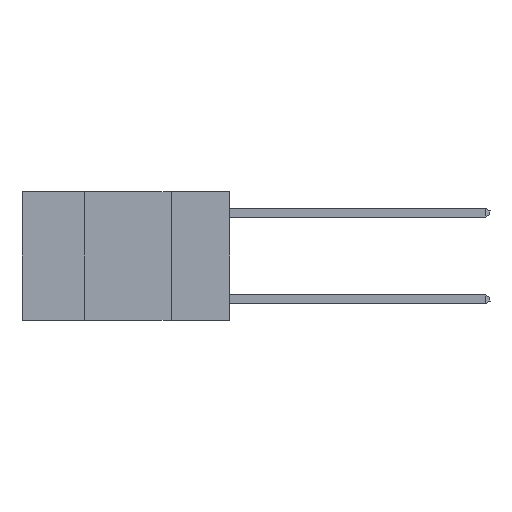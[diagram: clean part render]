
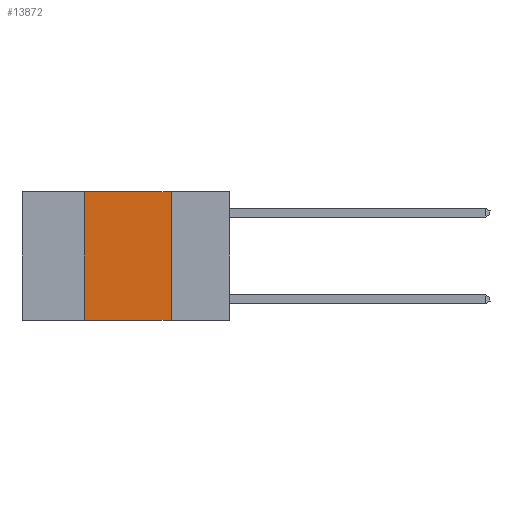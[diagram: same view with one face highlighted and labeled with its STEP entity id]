
A CAD part, left-side view. The second image highlights one B-rep face of the part: STEP entity #13872.
In plain terms, the highlighted planar face has unit normal (-1, 0, 0).
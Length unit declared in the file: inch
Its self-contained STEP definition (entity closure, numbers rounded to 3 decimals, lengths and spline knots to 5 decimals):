
#775 = CARTESIAN_POINT ( 'NONE',  ( 0., 0.17, 0. ) ) ;
#1298 = DIRECTION ( 'NONE',  ( 0., -1., 0. ) ) ;
#1736 = AXIS2_PLACEMENT_3D ( 'NONE', #2767, #10502, #3893 ) ;
#1818 = ORIENTED_EDGE ( 'NONE', *, *, #5294, .F. ) ;
#1974 = EDGE_CURVE ( 'NONE', #2466, #11475, #11461, .T. ) ;
#2466 = VERTEX_POINT ( 'NONE', #9969 ) ;
#2500 = CARTESIAN_POINT ( 'NONE',  ( 0., 0.6, 0. ) ) ;
#2698 = EDGE_CURVE ( 'NONE', #2466, #8263, #5739, .T. ) ;
#2767 = CARTESIAN_POINT ( 'NONE',  ( 0., 0.6, 0. ) ) ;
#3893 = DIRECTION ( 'NONE',  ( 0., 0., -1. ) ) ;
#4189 = EDGE_CURVE ( 'NONE', #6738, #11475, #9706, .T. ) ;
#4390 = FACE_OUTER_BOUND ( 'NONE', #12707, .T. ) ;
#4478 = CARTESIAN_POINT ( 'NONE',  ( 0., 0.42, 0. ) ) ;
#5294 = EDGE_CURVE ( 'NONE', #8263, #6738, #6561, .T. ) ;
#5739 = LINE ( 'NONE', #11353, #8341 ) ;
#6423 = VECTOR ( 'NONE', #12860, 39.37008 ) ;
#6561 = LINE ( 'NONE', #2500, #12085 ) ;
#6738 = VERTEX_POINT ( 'NONE', #10698 ) ;
#6791 = CARTESIAN_POINT ( 'NONE',  ( 0., 0.6, -0.37 ) ) ;
#8063 = DIRECTION ( 'NONE',  ( 0., -1., 0. ) ) ;
#8263 = VERTEX_POINT ( 'NONE', #4478 ) ;
#8341 = VECTOR ( 'NONE', #13511, 39.37008 ) ;
#8463 = CARTESIAN_POINT ( 'NONE',  ( 0., 0.17, -0.37 ) ) ;
#8531 = VECTOR ( 'NONE', #1298, 39.37008 ) ;
#9706 = LINE ( 'NONE', #775, #6423 ) ;
#9969 = CARTESIAN_POINT ( 'NONE',  ( 0., 0.42, -0.37 ) ) ;
#10273 = ORIENTED_EDGE ( 'NONE', *, *, #4189, .F. ) ;
#10454 = PLANE ( 'NONE',  #1736 ) ;
#10502 = DIRECTION ( 'NONE',  ( 1., 0., 0. ) ) ;
#10619 = ORIENTED_EDGE ( 'NONE', *, *, #2698, .F. ) ;
#10698 = CARTESIAN_POINT ( 'NONE',  ( 0., 0.17, 0. ) ) ;
#11353 = CARTESIAN_POINT ( 'NONE',  ( 0., 0.42, 0. ) ) ;
#11461 = LINE ( 'NONE', #6791, #8531 ) ;
#11475 = VERTEX_POINT ( 'NONE', #8463 ) ;
#12085 = VECTOR ( 'NONE', #8063, 39.37008 ) ;
#12707 = EDGE_LOOP ( 'NONE', ( #10273, #1818, #10619, #13531 ) ) ;
#12860 = DIRECTION ( 'NONE',  ( 0., 0., -1. ) ) ;
#13511 = DIRECTION ( 'NONE',  ( 0., 0., 1. ) ) ;
#13531 = ORIENTED_EDGE ( 'NONE', *, *, #1974, .T. ) ;
#13872 = ADVANCED_FACE ( 'NONE', ( #4390 ), #10454, .F. ) ;
